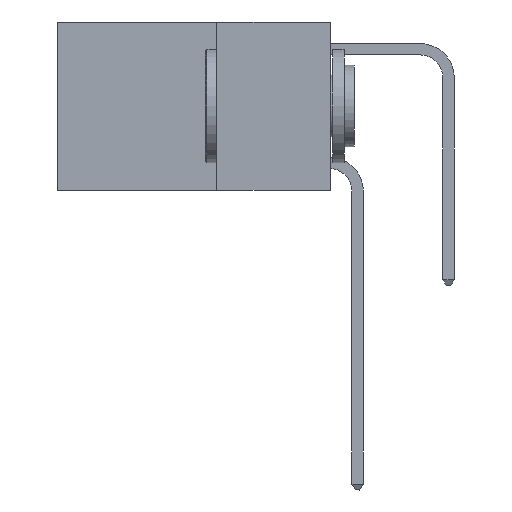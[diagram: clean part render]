
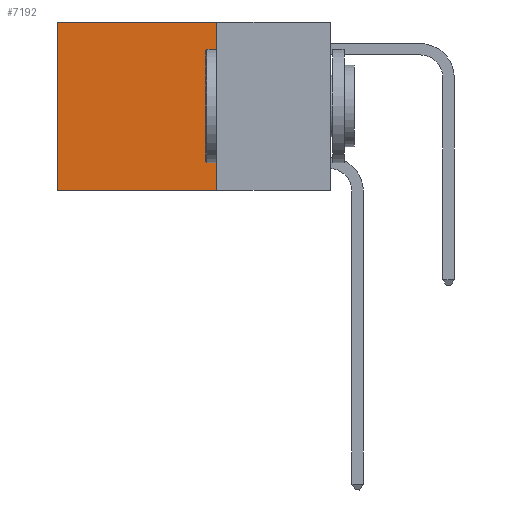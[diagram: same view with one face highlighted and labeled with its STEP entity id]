
A CAD part, left-side view. The second image highlights one B-rep face of the part: STEP entity #7192.
In plain terms, the highlighted planar face has unit normal (-1, 0, 0).
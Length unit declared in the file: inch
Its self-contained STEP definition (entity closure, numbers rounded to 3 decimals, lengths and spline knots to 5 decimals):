
#51 = VERTEX_POINT ( 'NONE', #5657 ) ;
#1040 = LINE ( 'NONE', #8735, #5869 ) ;
#1436 = DIRECTION ( 'NONE',  ( 0., 0., -1. ) ) ;
#1610 = CARTESIAN_POINT ( 'NONE',  ( 0.2625, 0.25, 0. ) ) ;
#1683 = VECTOR ( 'NONE', #3145, 39.37008 ) ;
#1846 = DIRECTION ( 'NONE',  ( 0., 0., -1. ) ) ;
#1901 = EDGE_CURVE ( 'NONE', #10598, #51, #1040, .T. ) ;
#2138 = EDGE_CURVE ( 'NONE', #10795, #4068, #10495, .T. ) ;
#3145 = DIRECTION ( 'NONE',  ( 0., 1., 0. ) ) ;
#3893 = ORIENTED_EDGE ( 'NONE', *, *, #2138, .F. ) ;
#4068 = VERTEX_POINT ( 'NONE', #8129 ) ;
#4144 = LINE ( 'NONE', #11129, #1683 ) ;
#4520 = CARTESIAN_POINT ( 'NONE',  ( 0.2625, 0.25, -0.37 ) ) ;
#4577 = CARTESIAN_POINT ( 'NONE',  ( 0.2625, 0.25, 0. ) ) ;
#4608 = LINE ( 'NONE', #4520, #9026 ) ;
#4642 = FACE_OUTER_BOUND ( 'NONE', #7410, .T. ) ;
#4985 = EDGE_CURVE ( 'NONE', #10795, #10598, #4144, .T. ) ;
#5657 = CARTESIAN_POINT ( 'NONE',  ( 0.2625, 0.6, -0.37 ) ) ;
#5746 = VECTOR ( 'NONE', #1436, 39.37008 ) ;
#5869 = VECTOR ( 'NONE', #8438, 39.37008 ) ;
#7185 = DIRECTION ( 'NONE',  ( 1., 0., 0. ) ) ;
#7192 = ADVANCED_FACE ( 'NONE', ( #4642 ), #8973, .F. ) ;
#7332 = ORIENTED_EDGE ( 'NONE', *, *, #4985, .T. ) ;
#7410 = EDGE_LOOP ( 'NONE', ( #9210, #9150, #3893, #7332 ) ) ;
#8129 = CARTESIAN_POINT ( 'NONE',  ( 0.2625, 0.25, -0.37 ) ) ;
#8438 = DIRECTION ( 'NONE',  ( 0., 0., -1. ) ) ;
#8615 = EDGE_CURVE ( 'NONE', #4068, #51, #4608, .T. ) ;
#8735 = CARTESIAN_POINT ( 'NONE',  ( 0.2625, 0.6, 0. ) ) ;
#8973 = PLANE ( 'NONE',  #9566 ) ;
#9026 = VECTOR ( 'NONE', #9839, 39.37008 ) ;
#9150 = ORIENTED_EDGE ( 'NONE', *, *, #8615, .F. ) ;
#9210 = ORIENTED_EDGE ( 'NONE', *, *, #1901, .T. ) ;
#9566 = AXIS2_PLACEMENT_3D ( 'NONE', #4577, #7185, #1846 ) ;
#9839 = DIRECTION ( 'NONE',  ( 0., 1., 0. ) ) ;
#10495 = LINE ( 'NONE', #1610, #5746 ) ;
#10598 = VERTEX_POINT ( 'NONE', #11342 ) ;
#10795 = VERTEX_POINT ( 'NONE', #11601 ) ;
#11129 = CARTESIAN_POINT ( 'NONE',  ( 0.2625, 0.25, 0. ) ) ;
#11342 = CARTESIAN_POINT ( 'NONE',  ( 0.2625, 0.6, 0. ) ) ;
#11601 = CARTESIAN_POINT ( 'NONE',  ( 0.2625, 0.25, 0. ) ) ;
